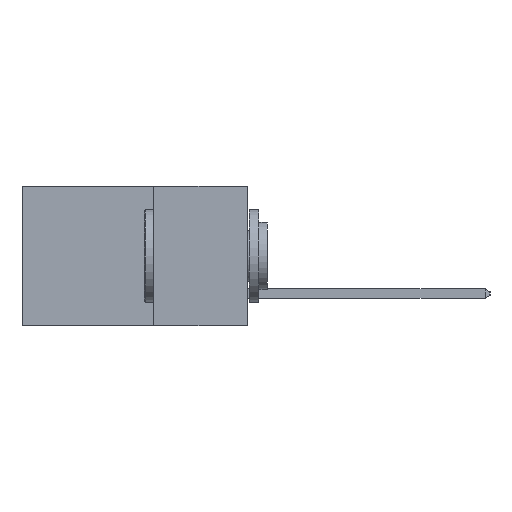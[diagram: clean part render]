
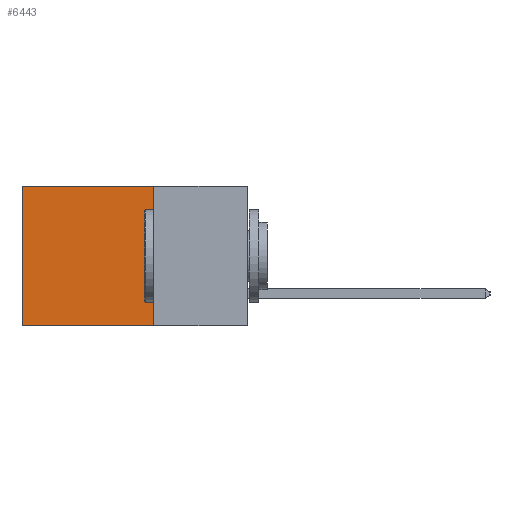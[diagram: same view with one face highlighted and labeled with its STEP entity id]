
A CAD part, left-side view. The second image highlights one B-rep face of the part: STEP entity #6443.
In plain terms, the highlighted planar face has unit normal (-1, 0, 0).
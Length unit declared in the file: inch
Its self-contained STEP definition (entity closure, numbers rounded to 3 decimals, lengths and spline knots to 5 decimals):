
#841 = LINE ( 'NONE', #3635, #11187 ) ;
#1135 = PLANE ( 'NONE',  #11409 ) ;
#1519 = LINE ( 'NONE', #11257, #10253 ) ;
#2399 = DIRECTION ( 'NONE',  ( 1., 0., 0. ) ) ;
#3635 = CARTESIAN_POINT ( 'NONE',  ( 0.2615, 0.25, -0.37 ) ) ;
#4496 = VECTOR ( 'NONE', #8534, 39.37008 ) ;
#4758 = DIRECTION ( 'NONE',  ( 0., 1., 0. ) ) ;
#5880 = VERTEX_POINT ( 'NONE', #7833 ) ;
#6106 = CARTESIAN_POINT ( 'NONE',  ( 0.2615, 0.25, 0. ) ) ;
#6426 = EDGE_CURVE ( 'NONE', #13957, #6473, #841, .T. ) ;
#6443 = ADVANCED_FACE ( 'NONE', ( #14248 ), #1135, .F. ) ;
#6473 = VERTEX_POINT ( 'NONE', #12799 ) ;
#6487 = EDGE_LOOP ( 'NONE', ( #13446, #13418, #13665, #13531 ) ) ;
#6891 = VERTEX_POINT ( 'NONE', #13594 ) ;
#7246 = CARTESIAN_POINT ( 'NONE',  ( 0.2615, 0.6, -0.37 ) ) ;
#7353 = LINE ( 'NONE', #7246, #13868 ) ;
#7833 = CARTESIAN_POINT ( 'NONE',  ( 0.2615, 0.6, -0.37 ) ) ;
#8534 = DIRECTION ( 'NONE',  ( 0., 1., 0. ) ) ;
#8574 = DIRECTION ( 'NONE',  ( 0., 0., -1. ) ) ;
#10207 = CARTESIAN_POINT ( 'NONE',  ( 0.2615, 0.25, -0.37 ) ) ;
#10253 = VECTOR ( 'NONE', #4758, 39.37008 ) ;
#10725 = EDGE_CURVE ( 'NONE', #6473, #5880, #11435, .T. ) ;
#11187 = VECTOR ( 'NONE', #14071, 39.37008 ) ;
#11257 = CARTESIAN_POINT ( 'NONE',  ( 0.2615, 0.25, 0. ) ) ;
#11394 = EDGE_CURVE ( 'NONE', #6891, #5880, #7353, .T. ) ;
#11409 = AXIS2_PLACEMENT_3D ( 'NONE', #10207, #2399, #11500 ) ;
#11435 = LINE ( 'NONE', #14947, #4496 ) ;
#11500 = DIRECTION ( 'NONE',  ( 0., 0., -1. ) ) ;
#12799 = CARTESIAN_POINT ( 'NONE',  ( 0.2615, 0.25, -0.37 ) ) ;
#13418 = ORIENTED_EDGE ( 'NONE', *, *, #10725, .F. ) ;
#13446 = ORIENTED_EDGE ( 'NONE', *, *, #11394, .T. ) ;
#13531 = ORIENTED_EDGE ( 'NONE', *, *, #13927, .T. ) ;
#13594 = CARTESIAN_POINT ( 'NONE',  ( 0.2615, 0.6, 0. ) ) ;
#13665 = ORIENTED_EDGE ( 'NONE', *, *, #6426, .F. ) ;
#13868 = VECTOR ( 'NONE', #8574, 39.37008 ) ;
#13927 = EDGE_CURVE ( 'NONE', #13957, #6891, #1519, .T. ) ;
#13957 = VERTEX_POINT ( 'NONE', #6106 ) ;
#14071 = DIRECTION ( 'NONE',  ( 0., 0., -1. ) ) ;
#14248 = FACE_OUTER_BOUND ( 'NONE', #6487, .T. ) ;
#14947 = CARTESIAN_POINT ( 'NONE',  ( 0.2615, 0.25, -0.37 ) ) ;
